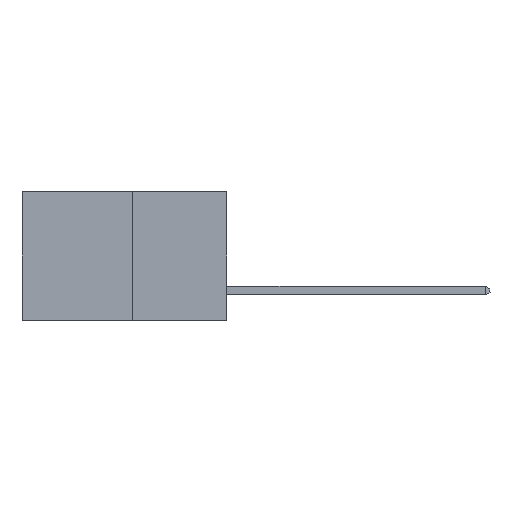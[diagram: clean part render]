
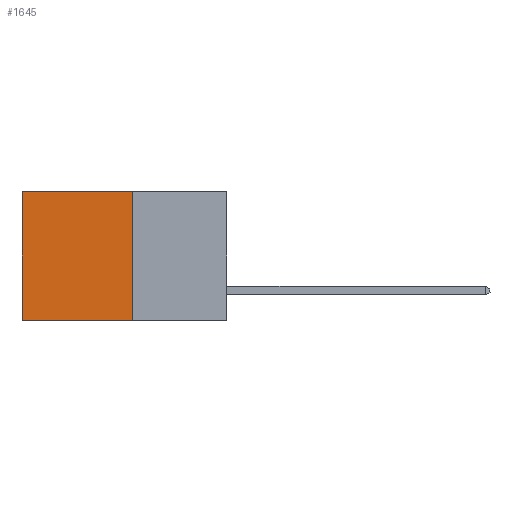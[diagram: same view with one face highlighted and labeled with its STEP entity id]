
A CAD part, left-side view. The second image highlights one B-rep face of the part: STEP entity #1645.
In plain terms, the highlighted planar face has unit normal (-1, 0, 0).
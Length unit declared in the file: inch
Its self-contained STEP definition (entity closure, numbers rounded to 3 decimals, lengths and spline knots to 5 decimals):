
#79 = ORIENTED_EDGE ( 'NONE', *, *, #316, .F. ) ;
#316 = EDGE_CURVE ( 'NONE', #1667, #1433, #8338, .T. ) ;
#404 = LINE ( 'NONE', #1112, #4134 ) ;
#418 = EDGE_LOOP ( 'NONE', ( #6971, #6512, #79, #6742 ) ) ;
#704 = FACE_OUTER_BOUND ( 'NONE', #418, .T. ) ;
#1007 = CARTESIAN_POINT ( 'NONE',  ( 0.277, 0.27, -0.37 ) ) ;
#1112 = CARTESIAN_POINT ( 'NONE',  ( 0.277, 0.59, -0.37 ) ) ;
#1157 = DIRECTION ( 'NONE',  ( 1., 0., 0. ) ) ;
#1166 = PLANE ( 'NONE',  #1789 ) ;
#1286 = LINE ( 'NONE', #4476, #8271 ) ;
#1366 = EDGE_CURVE ( 'NONE', #1667, #3860, #1286, .T. ) ;
#1433 = VERTEX_POINT ( 'NONE', #4819 ) ;
#1454 = VECTOR ( 'NONE', #4972, 39.37008 ) ;
#1645 = ADVANCED_FACE ( 'NONE', ( #704 ), #1166, .F. ) ;
#1667 = VERTEX_POINT ( 'NONE', #4914 ) ;
#1789 = AXIS2_PLACEMENT_3D ( 'NONE', #3106, #1157, #8300 ) ;
#2095 = CARTESIAN_POINT ( 'NONE',  ( 0.277, 0.59, -0.37 ) ) ;
#2802 = DIRECTION ( 'NONE',  ( 0., 0., -1. ) ) ;
#3106 = CARTESIAN_POINT ( 'NONE',  ( 0.277, 0.27, -0.37 ) ) ;
#3246 = DIRECTION ( 'NONE',  ( 0., 0., -1. ) ) ;
#3860 = VERTEX_POINT ( 'NONE', #7901 ) ;
#4134 = VECTOR ( 'NONE', #3246, 39.37008 ) ;
#4476 = CARTESIAN_POINT ( 'NONE',  ( 0.277, 0.27, 0. ) ) ;
#4600 = EDGE_CURVE ( 'NONE', #1433, #5160, #6920, .T. ) ;
#4819 = CARTESIAN_POINT ( 'NONE',  ( 0.277, 0.27, -0.37 ) ) ;
#4914 = CARTESIAN_POINT ( 'NONE',  ( 0.277, 0.27, 0. ) ) ;
#4972 = DIRECTION ( 'NONE',  ( 0., 1., 0. ) ) ;
#5160 = VERTEX_POINT ( 'NONE', #2095 ) ;
#5164 = CARTESIAN_POINT ( 'NONE',  ( 0.277, 0.27, -0.37 ) ) ;
#6512 = ORIENTED_EDGE ( 'NONE', *, *, #4600, .F. ) ;
#6742 = ORIENTED_EDGE ( 'NONE', *, *, #1366, .T. ) ;
#6767 = EDGE_CURVE ( 'NONE', #3860, #5160, #404, .T. ) ;
#6920 = LINE ( 'NONE', #5164, #1454 ) ;
#6971 = ORIENTED_EDGE ( 'NONE', *, *, #6767, .T. ) ;
#7901 = CARTESIAN_POINT ( 'NONE',  ( 0.277, 0.59, 0. ) ) ;
#7942 = DIRECTION ( 'NONE',  ( 0., 1., 0. ) ) ;
#8145 = VECTOR ( 'NONE', #2802, 39.37008 ) ;
#8271 = VECTOR ( 'NONE', #7942, 39.37008 ) ;
#8300 = DIRECTION ( 'NONE',  ( 0., 0., -1. ) ) ;
#8338 = LINE ( 'NONE', #1007, #8145 ) ;
